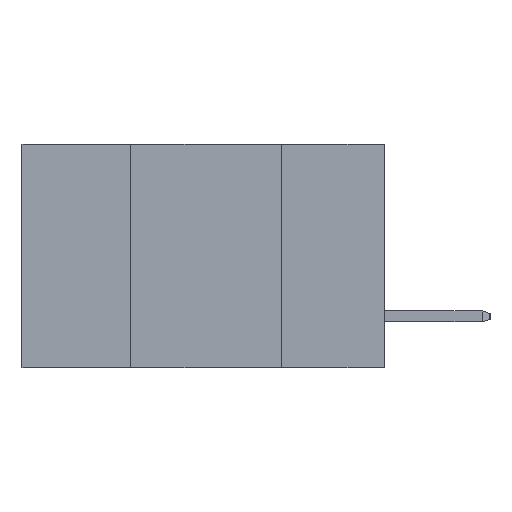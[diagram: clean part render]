
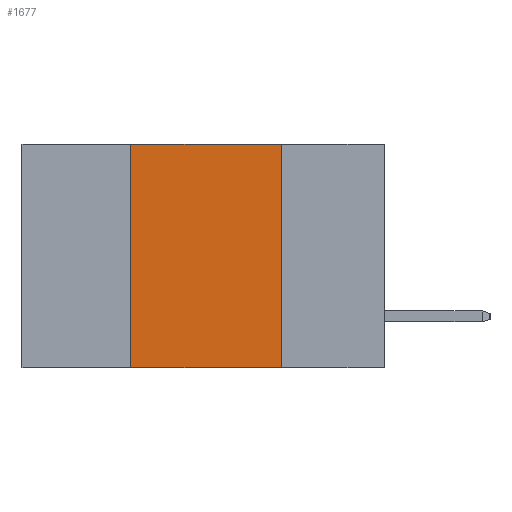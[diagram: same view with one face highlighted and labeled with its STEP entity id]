
A CAD part, left-side view. The second image highlights one B-rep face of the part: STEP entity #1677.
In plain terms, the highlighted planar face has unit normal (-1, 0, 0).
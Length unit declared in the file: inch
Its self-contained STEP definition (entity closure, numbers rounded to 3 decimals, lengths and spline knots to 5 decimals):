
#518 = CARTESIAN_POINT ( 'NONE',  ( 0., 0.17, -0.37 ) ) ;
#979 = EDGE_LOOP ( 'NONE', ( #12212, #11317, #15167, #11845 ) ) ;
#1042 = DIRECTION ( 'NONE',  ( 0., -1., 0. ) ) ;
#1124 = VECTOR ( 'NONE', #2757, 39.37008 ) ;
#1518 = VERTEX_POINT ( 'NONE', #5303 ) ;
#1677 = ADVANCED_FACE ( 'NONE', ( #15109 ), #3685, .F. ) ;
#2467 = LINE ( 'NONE', #13494, #8881 ) ;
#2757 = DIRECTION ( 'NONE',  ( 0., 0., 1. ) ) ;
#2844 = VECTOR ( 'NONE', #13647, 39.37008 ) ;
#3665 = DIRECTION ( 'NONE',  ( 1., 0., 0. ) ) ;
#3685 = PLANE ( 'NONE',  #3874 ) ;
#3874 = AXIS2_PLACEMENT_3D ( 'NONE', #10394, #3665, #4127 ) ;
#4127 = DIRECTION ( 'NONE',  ( 0., 0., -1. ) ) ;
#5303 = CARTESIAN_POINT ( 'NONE',  ( 0., 0.17, 0. ) ) ;
#6046 = VERTEX_POINT ( 'NONE', #518 ) ;
#6211 = VERTEX_POINT ( 'NONE', #15594 ) ;
#6294 = CARTESIAN_POINT ( 'NONE',  ( 0., 0.6, -0.37 ) ) ;
#7167 = VECTOR ( 'NONE', #7570, 39.37008 ) ;
#7190 = EDGE_CURVE ( 'NONE', #6211, #6046, #11983, .T. ) ;
#7570 = DIRECTION ( 'NONE',  ( 0., -1., 0. ) ) ;
#8048 = EDGE_CURVE ( 'NONE', #6211, #8112, #13999, .T. ) ;
#8112 = VERTEX_POINT ( 'NONE', #9234 ) ;
#8881 = VECTOR ( 'NONE', #1042, 39.37008 ) ;
#9234 = CARTESIAN_POINT ( 'NONE',  ( 0., 0.42, 0. ) ) ;
#9714 = EDGE_CURVE ( 'NONE', #8112, #1518, #2467, .T. ) ;
#10373 = CARTESIAN_POINT ( 'NONE',  ( 0., 0.42, -0.37 ) ) ;
#10394 = CARTESIAN_POINT ( 'NONE',  ( 0., 0.6, 0. ) ) ;
#11317 = ORIENTED_EDGE ( 'NONE', *, *, #9714, .F. ) ;
#11845 = ORIENTED_EDGE ( 'NONE', *, *, #7190, .T. ) ;
#11983 = LINE ( 'NONE', #6294, #7167 ) ;
#12130 = EDGE_CURVE ( 'NONE', #1518, #6046, #12824, .T. ) ;
#12212 = ORIENTED_EDGE ( 'NONE', *, *, #12130, .F. ) ;
#12460 = CARTESIAN_POINT ( 'NONE',  ( 0., 0.17, -0.37 ) ) ;
#12824 = LINE ( 'NONE', #12460, #2844 ) ;
#13494 = CARTESIAN_POINT ( 'NONE',  ( 0., 0.6, 0. ) ) ;
#13647 = DIRECTION ( 'NONE',  ( 0., 0., -1. ) ) ;
#13999 = LINE ( 'NONE', #10373, #1124 ) ;
#15109 = FACE_OUTER_BOUND ( 'NONE', #979, .T. ) ;
#15167 = ORIENTED_EDGE ( 'NONE', *, *, #8048, .F. ) ;
#15594 = CARTESIAN_POINT ( 'NONE',  ( 0., 0.42, -0.37 ) ) ;
